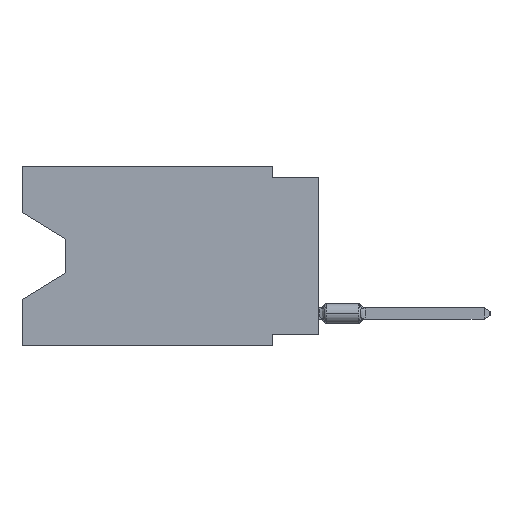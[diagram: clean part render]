
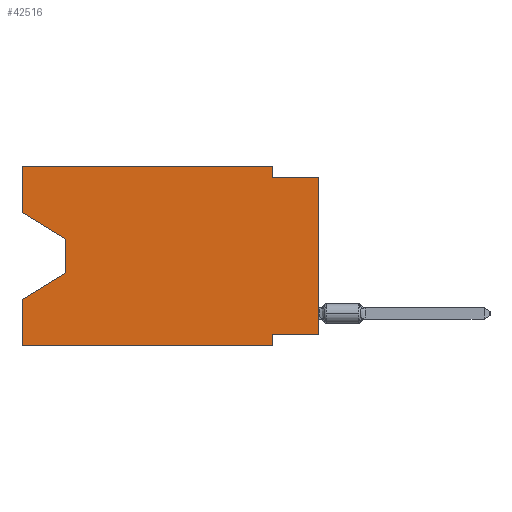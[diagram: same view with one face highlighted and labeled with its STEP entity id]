
A CAD part, left-side view. The second image highlights one B-rep face of the part: STEP entity #42516.
In plain terms, the highlighted planar face has unit normal (-1, 0, 0).
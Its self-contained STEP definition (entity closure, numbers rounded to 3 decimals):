
#448 = CARTESIAN_POINT ( 'NONE',  ( 0., 16.383, -2.546 ) ) ;
#842 = VERTEX_POINT ( 'NONE', #61736 ) ;
#5689 = LINE ( 'NONE', #49050, #34471 ) ;
#5939 = LINE ( 'NONE', #37948, #69725 ) ;
#6324 = ORIENTED_EDGE ( 'NONE', *, *, #29443, .T. ) ;
#6855 = CARTESIAN_POINT ( 'NONE',  ( 0., 13.97, -4.013 ) ) ;
#7116 = ORIENTED_EDGE ( 'NONE', *, *, #50775, .F. ) ;
#7945 = DIRECTION ( 'NONE',  ( 0., 0., -1. ) ) ;
#7994 = EDGE_CURVE ( 'NONE', #26040, #63318, #59345, .T. ) ;
#8551 = VECTOR ( 'NONE', #39637, 1000. ) ;
#9039 = PLANE ( 'NONE',  #21189 ) ;
#9117 = LINE ( 'NONE', #25117, #19796 ) ;
#9347 = EDGE_CURVE ( 'NONE', #842, #29766, #48153, .T. ) ;
#9522 = EDGE_CURVE ( 'NONE', #63318, #19127, #40288, .T. ) ;
#9547 = CARTESIAN_POINT ( 'NONE',  ( 0., 13.97, -4.013 ) ) ;
#9833 = DIRECTION ( 'NONE',  ( 0., -1., 0. ) ) ;
#10030 = ORIENTED_EDGE ( 'NONE', *, *, #27606, .F. ) ;
#10662 = ORIENTED_EDGE ( 'NONE', *, *, #9522, .F. ) ;
#10748 = ORIENTED_EDGE ( 'NONE', *, *, #68384, .F. ) ;
#10923 = VERTEX_POINT ( 'NONE', #56728 ) ;
#10929 = DIRECTION ( 'NONE',  ( 0., -1., 0. ) ) ;
#11263 = VECTOR ( 'NONE', #9833, 1000. ) ;
#12287 = CARTESIAN_POINT ( 'NONE',  ( 0., 2.54, -9.906 ) ) ;
#15802 = ORIENTED_EDGE ( 'NONE', *, *, #9347, .F. ) ;
#16102 = CARTESIAN_POINT ( 'NONE',  ( 0., 2.54, 0. ) ) ;
#18710 = VECTOR ( 'NONE', #54330, 1000. ) ;
#19127 = VERTEX_POINT ( 'NONE', #12287 ) ;
#19796 = VECTOR ( 'NONE', #62807, 1000. ) ;
#20068 = CARTESIAN_POINT ( 'NONE',  ( 0., 16.383, -9.906 ) ) ;
#20724 = CARTESIAN_POINT ( 'NONE',  ( 0., 16.383, 0. ) ) ;
#21189 = AXIS2_PLACEMENT_3D ( 'NONE', #20724, #30384, #58096 ) ;
#24504 = VECTOR ( 'NONE', #7945, 1000. ) ;
#25117 = CARTESIAN_POINT ( 'NONE',  ( 0., 0., 0. ) ) ;
#25192 = VERTEX_POINT ( 'NONE', #448 ) ;
#25883 = LINE ( 'NONE', #9547, #46057 ) ;
#25894 = CARTESIAN_POINT ( 'NONE',  ( 0., 16.383, 0. ) ) ;
#26040 = VERTEX_POINT ( 'NONE', #31761 ) ;
#27094 = CARTESIAN_POINT ( 'NONE',  ( 0., 2.54, -9.271 ) ) ;
#27606 = EDGE_CURVE ( 'NONE', #39963, #10923, #5939, .T. ) ;
#27858 = EDGE_CURVE ( 'NONE', #26040, #10923, #9117, .T. ) ;
#28146 = EDGE_LOOP ( 'NONE', ( #54483, #6324, #69168, #10748, #31405, #10662, #46185, #38793, #10030, #40208, #15802, #7116 ) ) ;
#29443 = EDGE_CURVE ( 'NONE', #68620, #67627, #25883, .T. ) ;
#29506 = VECTOR ( 'NONE', #70164, 1000. ) ;
#29766 = VERTEX_POINT ( 'NONE', #64402 ) ;
#30384 = DIRECTION ( 'NONE',  ( 1., 0., 0. ) ) ;
#31405 = ORIENTED_EDGE ( 'NONE', *, *, #35936, .T. ) ;
#31761 = CARTESIAN_POINT ( 'NONE',  ( 0., 0., -9.271 ) ) ;
#32298 = CARTESIAN_POINT ( 'NONE',  ( 0., 16.383, -2.546 ) ) ;
#34471 = VECTOR ( 'NONE', #43364, 1000. ) ;
#34502 = EDGE_CURVE ( 'NONE', #29766, #39963, #43467, .T. ) ;
#34958 = CARTESIAN_POINT ( 'NONE',  ( 0., 2.54, -9.906 ) ) ;
#35936 = EDGE_CURVE ( 'NONE', #48269, #19127, #48920, .T. ) ;
#36911 = DIRECTION ( 'NONE',  ( 0., 0., 1. ) ) ;
#37948 = CARTESIAN_POINT ( 'NONE',  ( 0., 0., -0.635 ) ) ;
#38793 = ORIENTED_EDGE ( 'NONE', *, *, #27858, .T. ) ;
#39637 = DIRECTION ( 'NONE',  ( 0., 0.855, -0.519 ) ) ;
#39963 = VERTEX_POINT ( 'NONE', #41136 ) ;
#40208 = ORIENTED_EDGE ( 'NONE', *, *, #34502, .F. ) ;
#40288 = LINE ( 'NONE', #34958, #24504 ) ;
#40383 = VECTOR ( 'NONE', #54881, 1000. ) ;
#41136 = CARTESIAN_POINT ( 'NONE',  ( 0., 2.54, -0.635 ) ) ;
#42516 = ADVANCED_FACE ( 'NONE', ( #46725 ), #9039, .F. ) ;
#43364 = DIRECTION ( 'NONE',  ( 0., 0., 1. ) ) ;
#43467 = LINE ( 'NONE', #16102, #29506 ) ;
#45568 = VERTEX_POINT ( 'NONE', #58820 ) ;
#46057 = VECTOR ( 'NONE', #69274, 1000. ) ;
#46185 = ORIENTED_EDGE ( 'NONE', *, *, #7994, .F. ) ;
#46725 = FACE_OUTER_BOUND ( 'NONE', #28146, .T. ) ;
#48153 = LINE ( 'NONE', #60232, #40383 ) ;
#48269 = VERTEX_POINT ( 'NONE', #20068 ) ;
#48920 = LINE ( 'NONE', #53558, #11263 ) ;
#49050 = CARTESIAN_POINT ( 'NONE',  ( 0., 16.383, 0. ) ) ;
#50775 = EDGE_CURVE ( 'NONE', #25192, #842, #5689, .T. ) ;
#53558 = CARTESIAN_POINT ( 'NONE',  ( 0., 16.383, -9.906 ) ) ;
#54330 = DIRECTION ( 'NONE',  ( 0., -0.855, -0.519 ) ) ;
#54483 = ORIENTED_EDGE ( 'NONE', *, *, #66901, .T. ) ;
#54498 = CARTESIAN_POINT ( 'NONE',  ( 0., 0., -9.271 ) ) ;
#54881 = DIRECTION ( 'NONE',  ( 0., -1., 0. ) ) ;
#56173 = VECTOR ( 'NONE', #68981, 1000. ) ;
#56410 = EDGE_CURVE ( 'NONE', #67627, #45568, #57662, .T. ) ;
#56728 = CARTESIAN_POINT ( 'NONE',  ( 0., 0., -0.635 ) ) ;
#57662 = LINE ( 'NONE', #67998, #8551 ) ;
#58096 = DIRECTION ( 'NONE',  ( 0., 0., -1. ) ) ;
#58820 = CARTESIAN_POINT ( 'NONE',  ( 0., 16.383, -7.36 ) ) ;
#59345 = LINE ( 'NONE', #54498, #56173 ) ;
#59622 = VECTOR ( 'NONE', #36911, 1000. ) ;
#60232 = CARTESIAN_POINT ( 'NONE',  ( 0., 16.383, 0. ) ) ;
#61736 = CARTESIAN_POINT ( 'NONE',  ( 0., 16.383, 0. ) ) ;
#62807 = DIRECTION ( 'NONE',  ( 0., 0., 1. ) ) ;
#63318 = VERTEX_POINT ( 'NONE', #27094 ) ;
#64402 = CARTESIAN_POINT ( 'NONE',  ( 0., 2.54, 0. ) ) ;
#64661 = LINE ( 'NONE', #32298, #18710 ) ;
#64998 = LINE ( 'NONE', #25894, #59622 ) ;
#66901 = EDGE_CURVE ( 'NONE', #25192, #68620, #64661, .T. ) ;
#67627 = VERTEX_POINT ( 'NONE', #67741 ) ;
#67741 = CARTESIAN_POINT ( 'NONE',  ( 0., 13.97, -5.893 ) ) ;
#67998 = CARTESIAN_POINT ( 'NONE',  ( 0., 13.97, -5.893 ) ) ;
#68384 = EDGE_CURVE ( 'NONE', #48269, #45568, #64998, .T. ) ;
#68620 = VERTEX_POINT ( 'NONE', #6855 ) ;
#68981 = DIRECTION ( 'NONE',  ( 0., 1., 0. ) ) ;
#69168 = ORIENTED_EDGE ( 'NONE', *, *, #56410, .T. ) ;
#69274 = DIRECTION ( 'NONE',  ( 0., 0., -1. ) ) ;
#69725 = VECTOR ( 'NONE', #10929, 1000. ) ;
#70164 = DIRECTION ( 'NONE',  ( 0., 0., -1. ) ) ;
